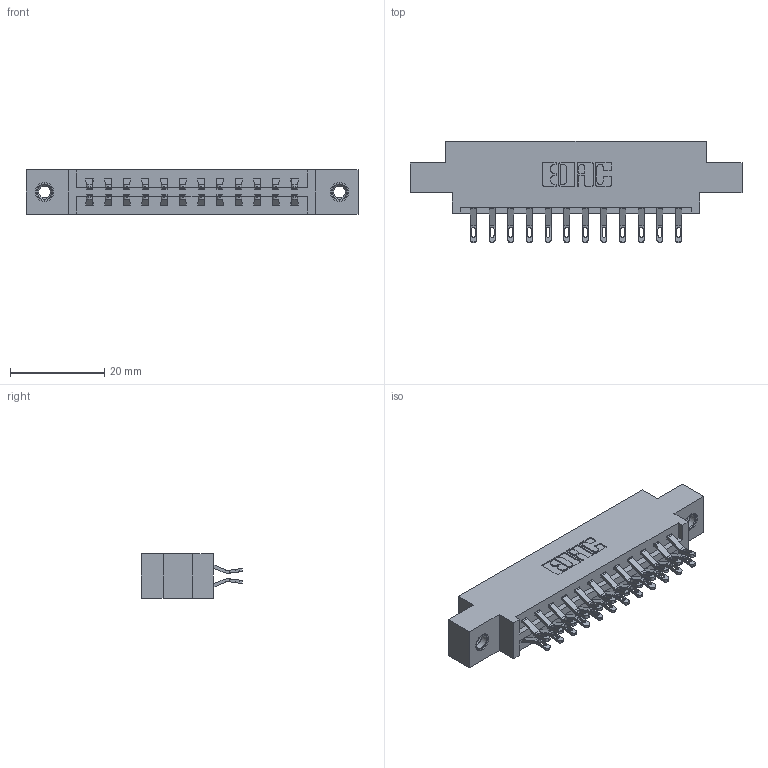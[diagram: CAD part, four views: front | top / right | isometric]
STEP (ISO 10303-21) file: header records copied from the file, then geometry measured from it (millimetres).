
FILE_DESCRIPTION (( 'STEP AP203' ), '1' );
FILE_NAME ('387-024-555-807.STEP', '2019-10-16T18:46:00', ( '' ), ( '' ), 'SwSTEP 2.0', 'SolidWorks 2016', '' );
FILE_SCHEMA (( 'CONFIG_CONTROL_DESIGN' ));
Length unit declared in the file: inch
Products named in the file (4): 345-292-001_555 Tail; 337 Part_0.170 Offset - 0.156 Dia-TI; 387-024-555-807; 345-250-001_345-250-005-103
Assembly tree (27 placements, depth 2):
  387-024-555-807
    337 Part_0.170 Offset - 0.156 Dia-TI
    345-292-001_555 Tail  x24
    345-250-001_345-250-005-103  x2
Bounding box: 70.56 x 21.47 x 9.4 mm (x, y, z)
Volume: 6975.6 mm3; surface area: 8000.6 mm2
Topology: 27 solids, 27 shells, 1618 faces, 4995 edges, 3322 vertices
Faces by surface type: plane 970, cylinder 632, cone 12, torus 4
Entity records: 14828 total; most frequent: CARTESIAN_POINT 2539, ORIENTED_EDGE 2438, DIRECTION 2217, EDGE_CURVE 1219, VECTOR 1051, LINE 1051, VERTEX_POINT 808, AXIS2_PLACEMENT_3D 583
